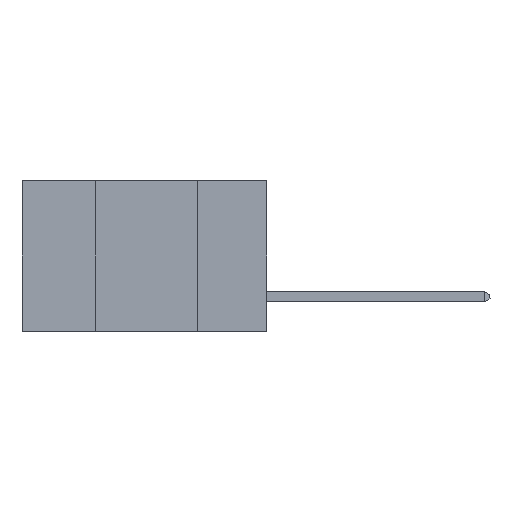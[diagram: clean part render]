
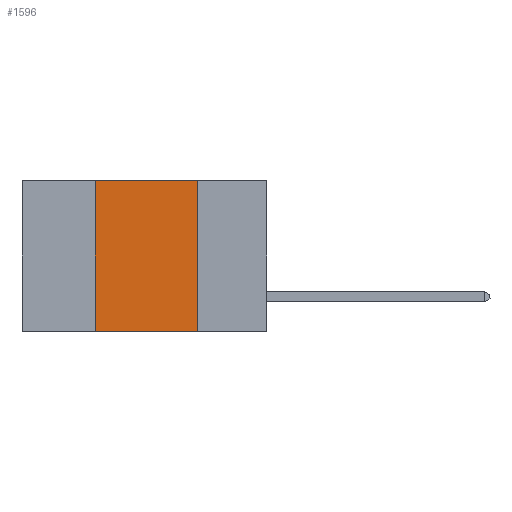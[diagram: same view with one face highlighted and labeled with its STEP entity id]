
A CAD part, left-side view. The second image highlights one B-rep face of the part: STEP entity #1596.
In plain terms, the highlighted planar face has unit normal (-1, 0, 0).
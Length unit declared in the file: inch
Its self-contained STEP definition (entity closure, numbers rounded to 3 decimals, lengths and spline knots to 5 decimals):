
#379 = VECTOR ( 'NONE', #2603, 39.37008 ) ;
#681 = LINE ( 'NONE', #2100, #379 ) ;
#864 = VECTOR ( 'NONE', #5690, 39.37008 ) ;
#1596 = ADVANCED_FACE ( 'NONE', ( #7806 ), #7963, .F. ) ;
#2017 = CARTESIAN_POINT ( 'NONE',  ( 0., 0.42, -0.37 ) ) ;
#2100 = CARTESIAN_POINT ( 'NONE',  ( 0., 0.17, 0. ) ) ;
#2570 = LINE ( 'NONE', #5227, #9259 ) ;
#2603 = DIRECTION ( 'NONE',  ( 0., 0., -1. ) ) ;
#2906 = VERTEX_POINT ( 'NONE', #9458 ) ;
#3821 = ORIENTED_EDGE ( 'NONE', *, *, #3909, .F. ) ;
#3862 = CARTESIAN_POINT ( 'NONE',  ( 0., 0.42, 0. ) ) ;
#3909 = EDGE_CURVE ( 'NONE', #2906, #8653, #681, .T. ) ;
#4644 = CARTESIAN_POINT ( 'NONE',  ( 0., 0.17, -0.37 ) ) ;
#4966 = DIRECTION ( 'NONE',  ( 0., -1., 0. ) ) ;
#5227 = CARTESIAN_POINT ( 'NONE',  ( 0., 0.6, 0. ) ) ;
#5544 = CARTESIAN_POINT ( 'NONE',  ( 0., 0.6, 0. ) ) ;
#5597 = AXIS2_PLACEMENT_3D ( 'NONE', #5544, #9497, #6132 ) ;
#5690 = DIRECTION ( 'NONE',  ( 0., 0., 1. ) ) ;
#6132 = DIRECTION ( 'NONE',  ( 0., 0., -1. ) ) ;
#6386 = EDGE_CURVE ( 'NONE', #11116, #2906, #2570, .T. ) ;
#6411 = CARTESIAN_POINT ( 'NONE',  ( 0., 0.42, 0. ) ) ;
#6446 = ORIENTED_EDGE ( 'NONE', *, *, #11214, .F. ) ;
#6704 = CARTESIAN_POINT ( 'NONE',  ( 0., 0.6, -0.37 ) ) ;
#6745 = DIRECTION ( 'NONE',  ( 0., -1., 0. ) ) ;
#7654 = ORIENTED_EDGE ( 'NONE', *, *, #6386, .F. ) ;
#7806 = FACE_OUTER_BOUND ( 'NONE', #9101, .T. ) ;
#7963 = PLANE ( 'NONE',  #5597 ) ;
#8058 = LINE ( 'NONE', #3862, #864 ) ;
#8653 = VERTEX_POINT ( 'NONE', #4644 ) ;
#9101 = EDGE_LOOP ( 'NONE', ( #3821, #7654, #6446, #10886 ) ) ;
#9259 = VECTOR ( 'NONE', #6745, 39.37008 ) ;
#9458 = CARTESIAN_POINT ( 'NONE',  ( 0., 0.17, 0. ) ) ;
#9490 = LINE ( 'NONE', #6704, #11348 ) ;
#9497 = DIRECTION ( 'NONE',  ( 1., 0., 0. ) ) ;
#10133 = EDGE_CURVE ( 'NONE', #11247, #8653, #9490, .T. ) ;
#10886 = ORIENTED_EDGE ( 'NONE', *, *, #10133, .T. ) ;
#11116 = VERTEX_POINT ( 'NONE', #6411 ) ;
#11214 = EDGE_CURVE ( 'NONE', #11247, #11116, #8058, .T. ) ;
#11247 = VERTEX_POINT ( 'NONE', #2017 ) ;
#11348 = VECTOR ( 'NONE', #4966, 39.37008 ) ;
